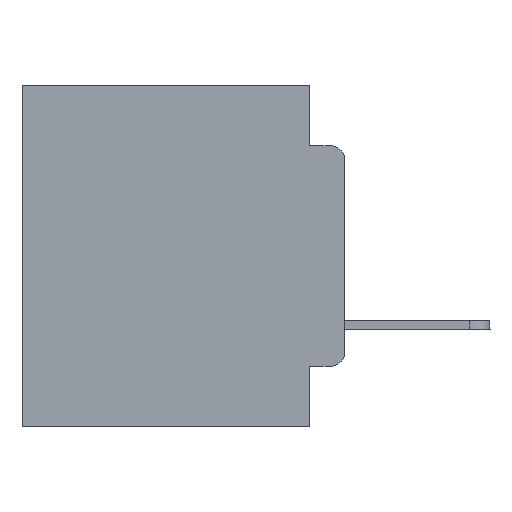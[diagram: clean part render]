
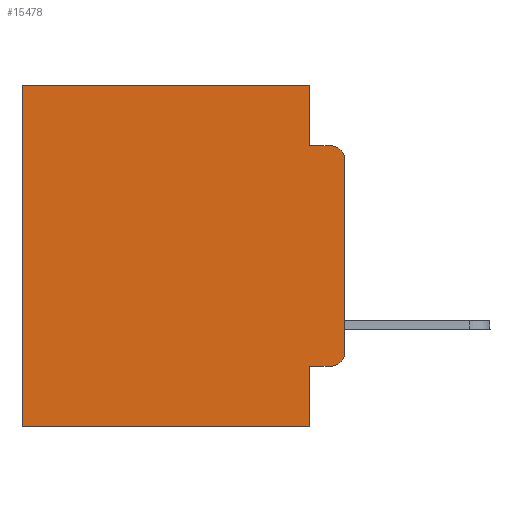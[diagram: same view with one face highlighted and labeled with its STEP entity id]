
A CAD part, left-side view. The second image highlights one B-rep face of the part: STEP entity #15478.
In plain terms, the highlighted planar face has unit normal (-1, 0, 0).
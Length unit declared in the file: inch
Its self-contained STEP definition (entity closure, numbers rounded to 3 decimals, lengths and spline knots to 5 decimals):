
#216 = EDGE_CURVE ( 'NONE', #23624, #26201, #20777, .T. ) ;
#676 = VERTEX_POINT ( 'NONE', #19763 ) ;
#2082 = AXIS2_PLACEMENT_3D ( 'NONE', #6770, #15343, #6919 ) ;
#2228 = DIRECTION ( 'NONE',  ( 0., 0., -1. ) ) ;
#2905 = ORIENTED_EDGE ( 'NONE', *, *, #21363, .T. ) ;
#3031 = CARTESIAN_POINT ( 'NONE',  ( 0.298, 0.051, -0.4115 ) ) ;
#3353 = DIRECTION ( 'NONE',  ( 0., 0., -1. ) ) ;
#3505 = CARTESIAN_POINT ( 'NONE',  ( 0.298, 0.051, 0. ) ) ;
#4027 = DIRECTION ( 'NONE',  ( 0., 1., 0. ) ) ;
#4101 = EDGE_LOOP ( 'NONE', ( #23157, #8795, #6672, #17793, #10913, #26829, #15846, #13833, #2905, #18324 ) ) ;
#4618 = LINE ( 'NONE', #10801, #26764 ) ;
#5152 = VERTEX_POINT ( 'NONE', #18725 ) ;
#5280 = DIRECTION ( 'NONE',  ( 0., 1., 0. ) ) ;
#5826 = EDGE_CURVE ( 'NONE', #26726, #14255, #26130, .T. ) ;
#6240 = DIRECTION ( 'NONE',  ( 0., 0., -1. ) ) ;
#6467 = EDGE_CURVE ( 'NONE', #676, #14255, #7947, .T. ) ;
#6672 = ORIENTED_EDGE ( 'NONE', *, *, #7776, .F. ) ;
#6708 = VERTEX_POINT ( 'NONE', #17054 ) ;
#6770 = CARTESIAN_POINT ( 'NONE',  ( 0.298, 0., 0. ) ) ;
#6919 = DIRECTION ( 'NONE',  ( 0., 0., -1. ) ) ;
#7035 = VECTOR ( 'NONE', #18673, 39.37008 ) ;
#7529 = LINE ( 'NONE', #3031, #25147 ) ;
#7588 = DIRECTION ( 'NONE',  ( 0., 0., -1. ) ) ;
#7776 = EDGE_CURVE ( 'NONE', #6708, #26523, #16748, .T. ) ;
#7947 = LINE ( 'NONE', #23123, #17182 ) ;
#8167 = CARTESIAN_POINT ( 'NONE',  ( 0.298, 0.051, -0.0885 ) ) ;
#8795 = ORIENTED_EDGE ( 'NONE', *, *, #18984, .T. ) ;
#8991 = DIRECTION ( 'NONE',  ( -1., 0., 0. ) ) ;
#9361 = CARTESIAN_POINT ( 'NONE',  ( 0.298, 0., -0.5 ) ) ;
#10251 = CARTESIAN_POINT ( 'NONE',  ( 0.298, 0.051, -0.5 ) ) ;
#10801 = CARTESIAN_POINT ( 'NONE',  ( 0.298, 0.473, 0. ) ) ;
#10913 = ORIENTED_EDGE ( 'NONE', *, *, #13262, .T. ) ;
#11782 = CARTESIAN_POINT ( 'NONE',  ( 0.298, 0.02, -0.1085 ) ) ;
#12058 = VECTOR ( 'NONE', #5280, 39.37008 ) ;
#13262 = EDGE_CURVE ( 'NONE', #24711, #22159, #23568, .T. ) ;
#13833 = ORIENTED_EDGE ( 'NONE', *, *, #216, .F. ) ;
#14255 = VERTEX_POINT ( 'NONE', #22357 ) ;
#15343 = DIRECTION ( 'NONE',  ( 1., 0., 0. ) ) ;
#15478 = ADVANCED_FACE ( 'NONE', ( #23771 ), #24058, .F. ) ;
#15846 = ORIENTED_EDGE ( 'NONE', *, *, #18261, .F. ) ;
#15981 = CARTESIAN_POINT ( 'NONE',  ( 0.298, 0.02, -0.0885 ) ) ;
#16173 = EDGE_CURVE ( 'NONE', #24711, #6708, #20368, .T. ) ;
#16396 = EDGE_CURVE ( 'NONE', #22159, #5152, #4618, .T. ) ;
#16470 = DIRECTION ( 'NONE',  ( 0., -1., 0. ) ) ;
#16748 = LINE ( 'NONE', #8167, #24442 ) ;
#17054 = CARTESIAN_POINT ( 'NONE',  ( 0.298, 0.051, -0.0885 ) ) ;
#17182 = VECTOR ( 'NONE', #6240, 39.37008 ) ;
#17545 = CARTESIAN_POINT ( 'NONE',  ( 0.298, 0.473, 0. ) ) ;
#17793 = ORIENTED_EDGE ( 'NONE', *, *, #16173, .F. ) ;
#18200 = DIRECTION ( 'NONE',  ( 0., -1., 0. ) ) ;
#18252 = CARTESIAN_POINT ( 'NONE',  ( 0.298, 0.051, 0. ) ) ;
#18261 = EDGE_CURVE ( 'NONE', #26201, #5152, #24535, .T. ) ;
#18324 = ORIENTED_EDGE ( 'NONE', *, *, #5826, .T. ) ;
#18536 = CARTESIAN_POINT ( 'NONE',  ( 0.298, 0.051, -0.4115 ) ) ;
#18673 = DIRECTION ( 'NONE',  ( 0., 0., -1. ) ) ;
#18725 = CARTESIAN_POINT ( 'NONE',  ( 0.298, 0.473, -0.5 ) ) ;
#18953 = AXIS2_PLACEMENT_3D ( 'NONE', #19512, #8991, #26113 ) ;
#18984 = EDGE_CURVE ( 'NONE', #676, #26523, #21065, .T. ) ;
#19512 = CARTESIAN_POINT ( 'NONE',  ( 0.298, 0.02, -0.3915 ) ) ;
#19763 = CARTESIAN_POINT ( 'NONE',  ( 0.298, 0., -0.1085 ) ) ;
#20368 = LINE ( 'NONE', #26813, #24996 ) ;
#20777 = LINE ( 'NONE', #3505, #7035 ) ;
#21065 = CIRCLE ( 'NONE', #25549, 0.02 ) ;
#21363 = EDGE_CURVE ( 'NONE', #23624, #26726, #7529, .T. ) ;
#21576 = CARTESIAN_POINT ( 'NONE',  ( 0.298, 0.02, -0.4115 ) ) ;
#22159 = VERTEX_POINT ( 'NONE', #17545 ) ;
#22172 = VECTOR ( 'NONE', #4027, 39.37008 ) ;
#22357 = CARTESIAN_POINT ( 'NONE',  ( 0.298, 0., -0.3915 ) ) ;
#22883 = DIRECTION ( 'NONE',  ( -1., 0., 0. ) ) ;
#23123 = CARTESIAN_POINT ( 'NONE',  ( 0.298, 0., 0. ) ) ;
#23157 = ORIENTED_EDGE ( 'NONE', *, *, #6467, .F. ) ;
#23285 = CARTESIAN_POINT ( 'NONE',  ( 0.298, 0., 0. ) ) ;
#23568 = LINE ( 'NONE', #23285, #22172 ) ;
#23624 = VERTEX_POINT ( 'NONE', #18536 ) ;
#23771 = FACE_OUTER_BOUND ( 'NONE', #4101, .T. ) ;
#24058 = PLANE ( 'NONE',  #2082 ) ;
#24442 = VECTOR ( 'NONE', #16470, 39.37008 ) ;
#24535 = LINE ( 'NONE', #9361, #12058 ) ;
#24711 = VERTEX_POINT ( 'NONE', #18252 ) ;
#24996 = VECTOR ( 'NONE', #7588, 39.37008 ) ;
#25147 = VECTOR ( 'NONE', #18200, 39.37008 ) ;
#25549 = AXIS2_PLACEMENT_3D ( 'NONE', #11782, #22883, #3353 ) ;
#26113 = DIRECTION ( 'NONE',  ( 0., 0., -1. ) ) ;
#26130 = CIRCLE ( 'NONE', #18953, 0.02 ) ;
#26201 = VERTEX_POINT ( 'NONE', #10251 ) ;
#26523 = VERTEX_POINT ( 'NONE', #15981 ) ;
#26726 = VERTEX_POINT ( 'NONE', #21576 ) ;
#26764 = VECTOR ( 'NONE', #2228, 39.37008 ) ;
#26813 = CARTESIAN_POINT ( 'NONE',  ( 0.298, 0.051, 0. ) ) ;
#26829 = ORIENTED_EDGE ( 'NONE', *, *, #16396, .T. ) ;
